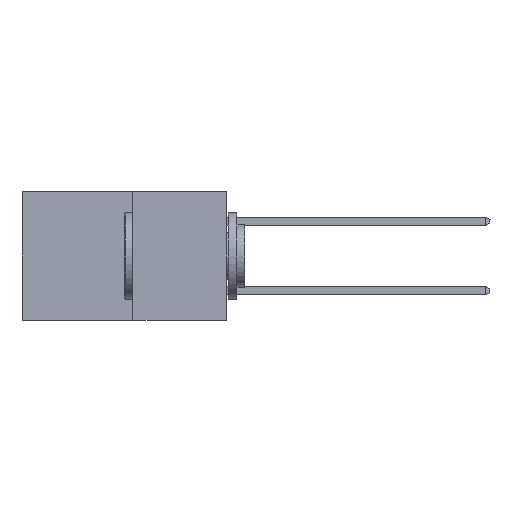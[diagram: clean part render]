
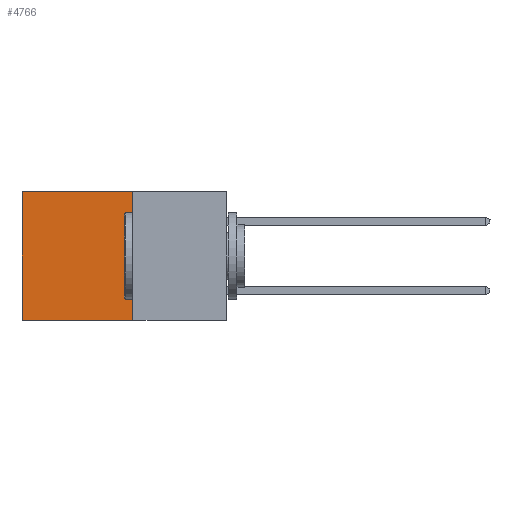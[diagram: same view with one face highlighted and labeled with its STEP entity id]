
A CAD part, left-side view. The second image highlights one B-rep face of the part: STEP entity #4766.
In plain terms, the highlighted planar face has unit normal (-1, 0, 0).
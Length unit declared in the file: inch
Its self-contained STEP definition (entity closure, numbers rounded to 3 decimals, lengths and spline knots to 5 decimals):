
#531 = DIRECTION ( 'NONE',  ( 0., 0., -1. ) ) ;
#1006 = CARTESIAN_POINT ( 'NONE',  ( 0.277, 0.59, -0.37 ) ) ;
#1007 = ORIENTED_EDGE ( 'NONE', *, *, #10340, .T. ) ;
#1632 = PLANE ( 'NONE',  #12937 ) ;
#2531 = VECTOR ( 'NONE', #9209, 39.37008 ) ;
#2933 = ORIENTED_EDGE ( 'NONE', *, *, #8868, .T. ) ;
#3044 = VECTOR ( 'NONE', #4792, 39.37008 ) ;
#3254 = VERTEX_POINT ( 'NONE', #4423 ) ;
#3756 = LINE ( 'NONE', #11860, #8222 ) ;
#3840 = VERTEX_POINT ( 'NONE', #5778 ) ;
#4423 = CARTESIAN_POINT ( 'NONE',  ( 0.277, 0.27, -0.37 ) ) ;
#4766 = ADVANCED_FACE ( 'NONE', ( #9173 ), #1632, .F. ) ;
#4792 = DIRECTION ( 'NONE',  ( 0., 1., 0. ) ) ;
#4848 = EDGE_CURVE ( 'NONE', #3840, #3254, #3756, .T. ) ;
#5026 = CARTESIAN_POINT ( 'NONE',  ( 0.277, 0.27, -0.37 ) ) ;
#5283 = LINE ( 'NONE', #1006, #2531 ) ;
#5509 = CARTESIAN_POINT ( 'NONE',  ( 0.277, 0.27, -0.37 ) ) ;
#5620 = ORIENTED_EDGE ( 'NONE', *, *, #4848, .F. ) ;
#5778 = CARTESIAN_POINT ( 'NONE',  ( 0.277, 0.27, 0. ) ) ;
#6847 = CARTESIAN_POINT ( 'NONE',  ( 0.277, 0.27, 0. ) ) ;
#7037 = CARTESIAN_POINT ( 'NONE',  ( 0.277, 0.59, 0. ) ) ;
#8186 = ORIENTED_EDGE ( 'NONE', *, *, #9602, .F. ) ;
#8222 = VECTOR ( 'NONE', #11728, 39.37008 ) ;
#8868 = EDGE_CURVE ( 'NONE', #3840, #10653, #11196, .T. ) ;
#9173 = FACE_OUTER_BOUND ( 'NONE', #9953, .T. ) ;
#9209 = DIRECTION ( 'NONE',  ( 0., 0., -1. ) ) ;
#9602 = EDGE_CURVE ( 'NONE', #3254, #11100, #10301, .T. ) ;
#9678 = CARTESIAN_POINT ( 'NONE',  ( 0.277, 0.59, -0.37 ) ) ;
#9953 = EDGE_LOOP ( 'NONE', ( #1007, #8186, #5620, #2933 ) ) ;
#9978 = VECTOR ( 'NONE', #13046, 39.37008 ) ;
#10301 = LINE ( 'NONE', #5026, #9978 ) ;
#10340 = EDGE_CURVE ( 'NONE', #10653, #11100, #5283, .T. ) ;
#10653 = VERTEX_POINT ( 'NONE', #7037 ) ;
#11100 = VERTEX_POINT ( 'NONE', #9678 ) ;
#11196 = LINE ( 'NONE', #6847, #3044 ) ;
#11728 = DIRECTION ( 'NONE',  ( 0., 0., -1. ) ) ;
#11745 = DIRECTION ( 'NONE',  ( 1., 0., 0. ) ) ;
#11860 = CARTESIAN_POINT ( 'NONE',  ( 0.277, 0.27, -0.37 ) ) ;
#12937 = AXIS2_PLACEMENT_3D ( 'NONE', #5509, #11745, #531 ) ;
#13046 = DIRECTION ( 'NONE',  ( 0., 1., 0. ) ) ;
